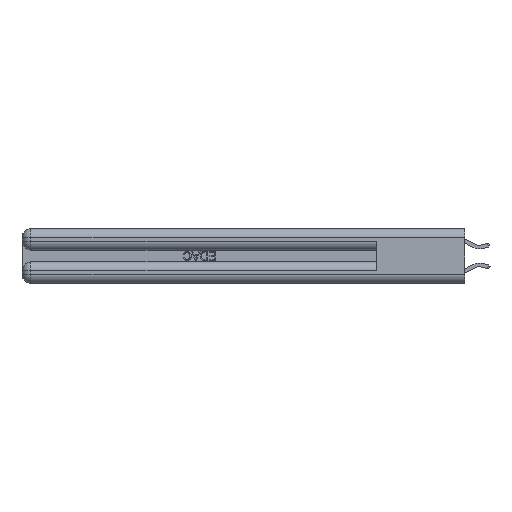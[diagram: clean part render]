
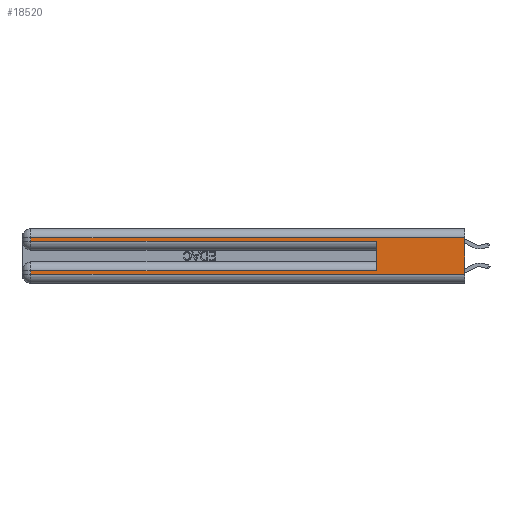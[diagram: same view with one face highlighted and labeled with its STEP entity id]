
A CAD part, left-side view. The second image highlights one B-rep face of the part: STEP entity #18520.
In plain terms, the highlighted planar face has unit normal (-1, 0, 0).
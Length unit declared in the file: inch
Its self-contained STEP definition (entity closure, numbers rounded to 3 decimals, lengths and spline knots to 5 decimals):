
#1588 = CARTESIAN_POINT ( 'NONE',  ( 0., 2.94, 0.31 ) ) ;
#1612 = CARTESIAN_POINT ( 'NONE',  ( 0., 0., 0.37 ) ) ;
#1986 = VERTEX_POINT ( 'NONE', #10768 ) ;
#2298 = CARTESIAN_POINT ( 'NONE',  ( 0., 0., 0.085 ) ) ;
#2569 = LINE ( 'NONE', #3116, #31419 ) ;
#2731 = LINE ( 'NONE', #29573, #17288 ) ;
#3116 = CARTESIAN_POINT ( 'NONE',  ( 0., 2.94, 0.37 ) ) ;
#4176 = CARTESIAN_POINT ( 'NONE',  ( 0., 0.6, 0.285 ) ) ;
#4248 = EDGE_CURVE ( 'NONE', #5813, #1986, #7692, .T. ) ;
#4699 = EDGE_CURVE ( 'NONE', #29325, #11116, #9910, .T. ) ;
#4753 = CARTESIAN_POINT ( 'NONE',  ( 0., 0., 0.31 ) ) ;
#5393 = EDGE_CURVE ( 'NONE', #29325, #11784, #7372, .T. ) ;
#5552 = DIRECTION ( 'NONE',  ( 0., 0., -1. ) ) ;
#5641 = VECTOR ( 'NONE', #7471, 39.37008 ) ;
#5813 = VERTEX_POINT ( 'NONE', #15501 ) ;
#6529 = EDGE_CURVE ( 'NONE', #11116, #12580, #19179, .T. ) ;
#7277 = PLANE ( 'NONE',  #24656 ) ;
#7372 = LINE ( 'NONE', #1612, #15819 ) ;
#7471 = DIRECTION ( 'NONE',  ( 0., 1., 0. ) ) ;
#7667 = LINE ( 'NONE', #18733, #23651 ) ;
#7692 = LINE ( 'NONE', #2298, #16952 ) ;
#8333 = CARTESIAN_POINT ( 'NONE',  ( 0., 0., 0.06 ) ) ;
#8868 = EDGE_CURVE ( 'NONE', #12580, #36255, #7667, .T. ) ;
#8886 = CARTESIAN_POINT ( 'NONE',  ( 0., 2.94, 0.37 ) ) ;
#9635 = EDGE_LOOP ( 'NONE', ( #35729, #26544, #14993, #15082, #10633, #22364, #30844, #18246 ) ) ;
#9668 = EDGE_CURVE ( 'NONE', #5813, #36255, #2731, .T. ) ;
#9910 = LINE ( 'NONE', #19078, #5641 ) ;
#10633 = ORIENTED_EDGE ( 'NONE', *, *, #9668, .F. ) ;
#10761 = CARTESIAN_POINT ( 'NONE',  ( 0., 2.94, 0.06 ) ) ;
#10768 = CARTESIAN_POINT ( 'NONE',  ( 0., 2.94, 0.085 ) ) ;
#11116 = VERTEX_POINT ( 'NONE', #1588 ) ;
#11784 = VERTEX_POINT ( 'NONE', #19429 ) ;
#12580 = VERTEX_POINT ( 'NONE', #35944 ) ;
#12872 = VECTOR ( 'NONE', #19760, 39.37008 ) ;
#14993 = ORIENTED_EDGE ( 'NONE', *, *, #6529, .T. ) ;
#15082 = ORIENTED_EDGE ( 'NONE', *, *, #8868, .T. ) ;
#15501 = CARTESIAN_POINT ( 'NONE',  ( 0., 0.6, 0.085 ) ) ;
#15819 = VECTOR ( 'NONE', #30567, 39.37008 ) ;
#16051 = DIRECTION ( 'NONE',  ( 0., 0., -1. ) ) ;
#16296 = DIRECTION ( 'NONE',  ( 0., 1., 0. ) ) ;
#16952 = VECTOR ( 'NONE', #16296, 39.37008 ) ;
#17288 = VECTOR ( 'NONE', #32182, 39.37008 ) ;
#18246 = ORIENTED_EDGE ( 'NONE', *, *, #35798, .T. ) ;
#18520 = ADVANCED_FACE ( 'NONE', ( #33093 ), #7277, .F. ) ;
#18733 = CARTESIAN_POINT ( 'NONE',  ( 0., 0., 0.285 ) ) ;
#19078 = CARTESIAN_POINT ( 'NONE',  ( 0., 0., 0.31 ) ) ;
#19179 = LINE ( 'NONE', #8886, #29682 ) ;
#19429 = CARTESIAN_POINT ( 'NONE',  ( 0., 0., 0.06 ) ) ;
#19760 = DIRECTION ( 'NONE',  ( 0., -1., 0. ) ) ;
#22364 = ORIENTED_EDGE ( 'NONE', *, *, #4248, .T. ) ;
#23651 = VECTOR ( 'NONE', #27479, 39.37008 ) ;
#24656 = AXIS2_PLACEMENT_3D ( 'NONE', #29921, #30293, #16051 ) ;
#26544 = ORIENTED_EDGE ( 'NONE', *, *, #4699, .T. ) ;
#27479 = DIRECTION ( 'NONE',  ( 0., -1., 0. ) ) ;
#27700 = VERTEX_POINT ( 'NONE', #10761 ) ;
#28344 = DIRECTION ( 'NONE',  ( 0., 0., -1. ) ) ;
#29325 = VERTEX_POINT ( 'NONE', #4753 ) ;
#29573 = CARTESIAN_POINT ( 'NONE',  ( 0., 0.6, 0.145 ) ) ;
#29682 = VECTOR ( 'NONE', #28344, 39.37008 ) ;
#29921 = CARTESIAN_POINT ( 'NONE',  ( 0., 0., 0.37 ) ) ;
#30293 = DIRECTION ( 'NONE',  ( 1., 0., 0. ) ) ;
#30567 = DIRECTION ( 'NONE',  ( 0., 0., -1. ) ) ;
#30844 = ORIENTED_EDGE ( 'NONE', *, *, #34416, .T. ) ;
#31419 = VECTOR ( 'NONE', #5552, 39.37008 ) ;
#32182 = DIRECTION ( 'NONE',  ( 0., 0., 1. ) ) ;
#33093 = FACE_OUTER_BOUND ( 'NONE', #9635, .T. ) ;
#33965 = LINE ( 'NONE', #8333, #12872 ) ;
#34416 = EDGE_CURVE ( 'NONE', #1986, #27700, #2569, .T. ) ;
#35729 = ORIENTED_EDGE ( 'NONE', *, *, #5393, .F. ) ;
#35798 = EDGE_CURVE ( 'NONE', #27700, #11784, #33965, .T. ) ;
#35944 = CARTESIAN_POINT ( 'NONE',  ( 0., 2.94, 0.285 ) ) ;
#36255 = VERTEX_POINT ( 'NONE', #4176 ) ;
